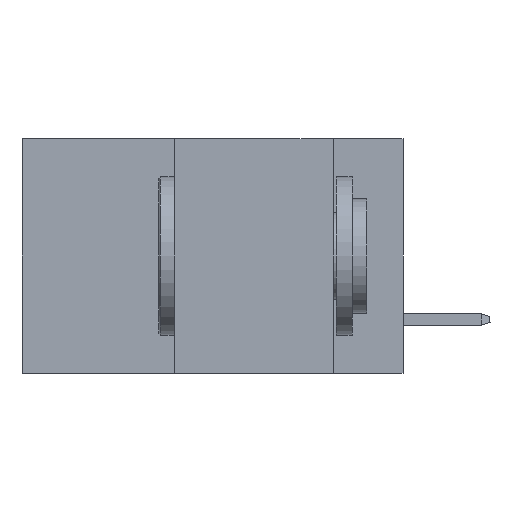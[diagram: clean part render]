
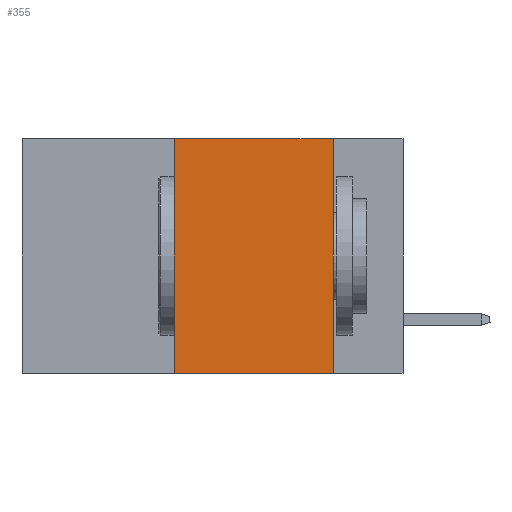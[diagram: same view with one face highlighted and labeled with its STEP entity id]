
A CAD part, left-side view. The second image highlights one B-rep face of the part: STEP entity #355.
In plain terms, the highlighted planar face has unit normal (-1, 0, 0).
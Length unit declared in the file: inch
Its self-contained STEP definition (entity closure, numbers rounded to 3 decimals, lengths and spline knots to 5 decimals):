
#355 = ADVANCED_FACE ( 'NONE', ( #36011 ), #22940, .F. ) ;
#373 = VERTEX_POINT ( 'NONE', #1433 ) ;
#847 = CARTESIAN_POINT ( 'NONE',  ( 0., 0.36, -0.37 ) ) ;
#1163 = VECTOR ( 'NONE', #7793, 39.37008 ) ;
#1433 = CARTESIAN_POINT ( 'NONE',  ( 0., 0.11, 0. ) ) ;
#1712 = VERTEX_POINT ( 'NONE', #39932 ) ;
#2025 = ORIENTED_EDGE ( 'NONE', *, *, #4835, .F. ) ;
#4835 = EDGE_CURVE ( 'NONE', #26920, #373, #17380, .T. ) ;
#5532 = VERTEX_POINT ( 'NONE', #847 ) ;
#7498 = CARTESIAN_POINT ( 'NONE',  ( 0., 0.6, 0. ) ) ;
#7793 = DIRECTION ( 'NONE',  ( 0., -1., 0. ) ) ;
#9003 = ORIENTED_EDGE ( 'NONE', *, *, #24514, .F. ) ;
#9725 = VECTOR ( 'NONE', #34817, 39.37008 ) ;
#11786 = LINE ( 'NONE', #18816, #9725 ) ;
#13130 = LINE ( 'NONE', #20130, #18342 ) ;
#15656 = EDGE_CURVE ( 'NONE', #373, #1712, #21244, .T. ) ;
#15957 = ORIENTED_EDGE ( 'NONE', *, *, #22704, .T. ) ;
#17380 = LINE ( 'NONE', #23642, #1163 ) ;
#18342 = VECTOR ( 'NONE', #32817, 39.37008 ) ;
#18816 = CARTESIAN_POINT ( 'NONE',  ( 0., 0.36, 0. ) ) ;
#19665 = ORIENTED_EDGE ( 'NONE', *, *, #15656, .F. ) ;
#20130 = CARTESIAN_POINT ( 'NONE',  ( 0., 0.6, -0.37 ) ) ;
#20199 = DIRECTION ( 'NONE',  ( 1., 0., 0. ) ) ;
#21244 = LINE ( 'NONE', #31434, #23038 ) ;
#22704 = EDGE_CURVE ( 'NONE', #5532, #1712, #13130, .T. ) ;
#22940 = PLANE ( 'NONE',  #29700 ) ;
#23038 = VECTOR ( 'NONE', #27700, 39.37008 ) ;
#23642 = CARTESIAN_POINT ( 'NONE',  ( 0., 0.6, 0. ) ) ;
#24514 = EDGE_CURVE ( 'NONE', #5532, #26920, #11786, .T. ) ;
#26920 = VERTEX_POINT ( 'NONE', #29563 ) ;
#27700 = DIRECTION ( 'NONE',  ( 0., 0., -1. ) ) ;
#28008 = EDGE_LOOP ( 'NONE', ( #19665, #2025, #9003, #15957 ) ) ;
#29563 = CARTESIAN_POINT ( 'NONE',  ( 0., 0.36, 0. ) ) ;
#29700 = AXIS2_PLACEMENT_3D ( 'NONE', #7498, #20199, #33090 ) ;
#31434 = CARTESIAN_POINT ( 'NONE',  ( 0., 0.11, 0. ) ) ;
#32817 = DIRECTION ( 'NONE',  ( 0., -1., 0. ) ) ;
#33090 = DIRECTION ( 'NONE',  ( 0., 0., -1. ) ) ;
#34817 = DIRECTION ( 'NONE',  ( 0., 0., 1. ) ) ;
#36011 = FACE_OUTER_BOUND ( 'NONE', #28008, .T. ) ;
#39932 = CARTESIAN_POINT ( 'NONE',  ( 0., 0.11, -0.37 ) ) ;
